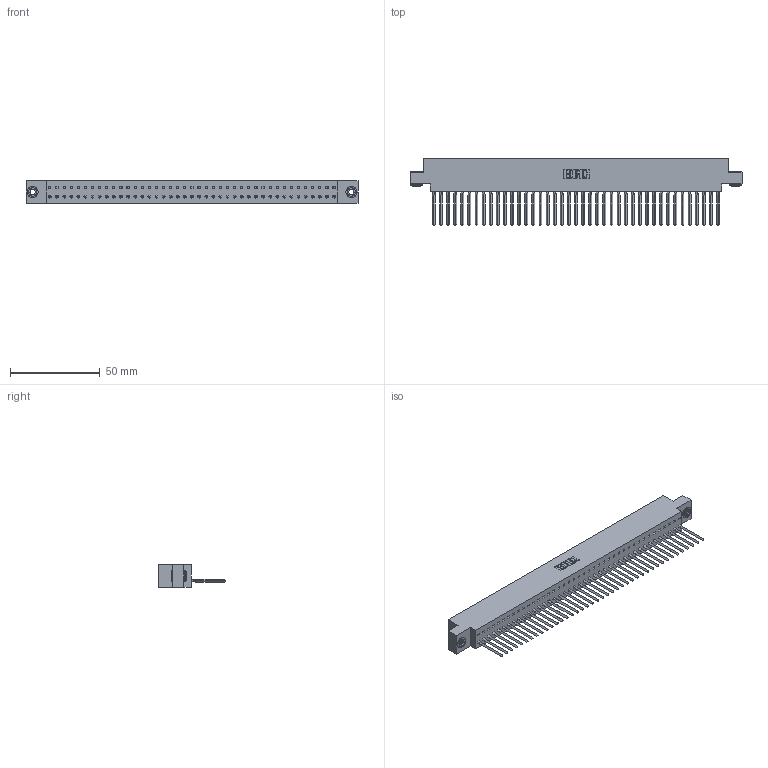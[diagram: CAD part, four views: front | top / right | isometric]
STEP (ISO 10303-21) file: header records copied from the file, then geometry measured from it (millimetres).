
FILE_DESCRIPTION (( 'STEP AP203' ), '1' );
FILE_NAME ('317-041-541-603.STEP', '2020-02-28T00:56:24', ( '' ), ( '' ), 'SwSTEP 2.0', 'SolidWorks 2016', '' );
FILE_SCHEMA (( 'CONFIG_CONTROL_DESIGN' ));
Length unit declared in the file: inch
Products named in the file (4): 317-041-541-603; 317-290-002_541; 345-250-002_345-250-002-102; 317 Part_.156 Dia - TH
Assembly tree (44 placements, depth 2):
  317-041-541-603
    317 Part_.156 Dia - TH
    317-290-002_541  x41
    345-250-002_345-250-002-102  x2
Bounding box: 185.17 x 37.34 x 12.7 mm (x, y, z)
Volume: 30016.4 mm3; surface area: 42596.5 mm2
Topology: 44 solids, 44 shells, 6372 faces, 18145 edges, 11792 vertices
Faces by surface type: plane 5152, cylinder 1048, bspline 164, cone 8
Entity records: 60291 total; most frequent: CARTESIAN_POINT 11327, ORIENTED_EDGE 10614, DIRECTION 8759, EDGE_CURVE 5307, LINE 4919, VECTOR 4919, VERTEX_POINT 3528, AXIS2_PLACEMENT_3D 1920
